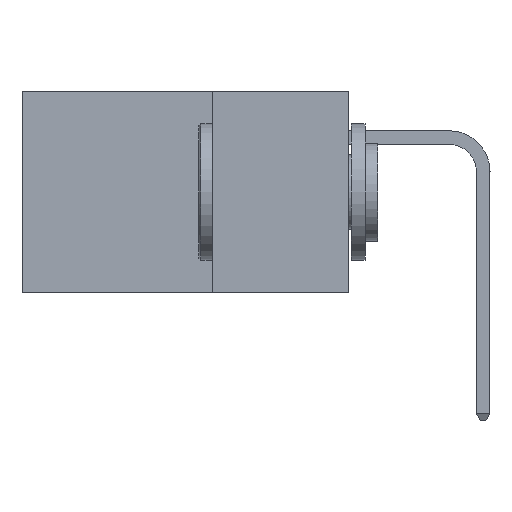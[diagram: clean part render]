
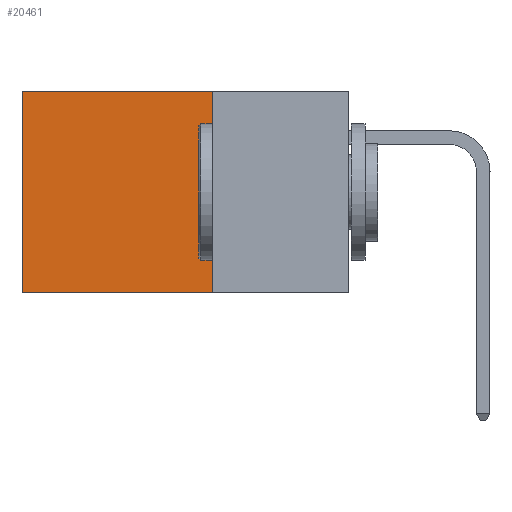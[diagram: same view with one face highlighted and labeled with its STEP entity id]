
A CAD part, left-side view. The second image highlights one B-rep face of the part: STEP entity #20461.
In plain terms, the highlighted planar face has unit normal (-1, 0, 0).
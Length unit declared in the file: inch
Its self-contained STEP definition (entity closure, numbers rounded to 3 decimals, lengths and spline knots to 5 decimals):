
#91 = ORIENTED_EDGE ( 'NONE', *, *, #22692, .F. ) ;
#174 = ORIENTED_EDGE ( 'NONE', *, *, #23511, .T. ) ;
#1200 = VECTOR ( 'NONE', #4552, 39.37008 ) ;
#3024 = VERTEX_POINT ( 'NONE', #3684 ) ;
#3476 = DIRECTION ( 'NONE',  ( 0., 0., -1. ) ) ;
#3684 = CARTESIAN_POINT ( 'NONE',  ( 0.2875, 0.6, 0. ) ) ;
#3872 = ORIENTED_EDGE ( 'NONE', *, *, #16571, .T. ) ;
#4496 = VERTEX_POINT ( 'NONE', #9836 ) ;
#4552 = DIRECTION ( 'NONE',  ( 0., 1., 0. ) ) ;
#5365 = VECTOR ( 'NONE', #17364, 39.37008 ) ;
#6536 = LINE ( 'NONE', #16033, #11114 ) ;
#7204 = EDGE_CURVE ( 'NONE', #16141, #8406, #10512, .T. ) ;
#8406 = VERTEX_POINT ( 'NONE', #18726 ) ;
#9836 = CARTESIAN_POINT ( 'NONE',  ( 0.2875, 0.6, -0.37 ) ) ;
#10512 = LINE ( 'NONE', #13043, #25504 ) ;
#11114 = VECTOR ( 'NONE', #19956, 39.37008 ) ;
#11266 = PLANE ( 'NONE',  #23956 ) ;
#12332 = LINE ( 'NONE', #24047, #1200 ) ;
#12770 = ORIENTED_EDGE ( 'NONE', *, *, #7204, .F. ) ;
#13043 = CARTESIAN_POINT ( 'NONE',  ( 0.2875, 0.25, 0. ) ) ;
#13286 = CARTESIAN_POINT ( 'NONE',  ( 0.2875, 0.25, 0. ) ) ;
#15019 = DIRECTION ( 'NONE',  ( 0., 0., -1. ) ) ;
#15235 = DIRECTION ( 'NONE',  ( 1., 0., 0. ) ) ;
#15407 = CARTESIAN_POINT ( 'NONE',  ( 0.2875, 0.25, -0.37 ) ) ;
#16033 = CARTESIAN_POINT ( 'NONE',  ( 0.2875, 0.6, 0. ) ) ;
#16141 = VERTEX_POINT ( 'NONE', #16624 ) ;
#16178 = EDGE_LOOP ( 'NONE', ( #174, #91, #12770, #3872 ) ) ;
#16571 = EDGE_CURVE ( 'NONE', #16141, #3024, #12332, .T. ) ;
#16624 = CARTESIAN_POINT ( 'NONE',  ( 0.2875, 0.25, 0. ) ) ;
#17364 = DIRECTION ( 'NONE',  ( 0., 1., 0. ) ) ;
#18726 = CARTESIAN_POINT ( 'NONE',  ( 0.2875, 0.25, -0.37 ) ) ;
#19956 = DIRECTION ( 'NONE',  ( 0., 0., -1. ) ) ;
#20436 = FACE_OUTER_BOUND ( 'NONE', #16178, .T. ) ;
#20461 = ADVANCED_FACE ( 'NONE', ( #20436 ), #11266, .F. ) ;
#21021 = LINE ( 'NONE', #15407, #5365 ) ;
#22692 = EDGE_CURVE ( 'NONE', #8406, #4496, #21021, .T. ) ;
#23511 = EDGE_CURVE ( 'NONE', #3024, #4496, #6536, .T. ) ;
#23956 = AXIS2_PLACEMENT_3D ( 'NONE', #13286, #15235, #3476 ) ;
#24047 = CARTESIAN_POINT ( 'NONE',  ( 0.2875, 0.25, 0. ) ) ;
#25504 = VECTOR ( 'NONE', #15019, 39.37008 ) ;
